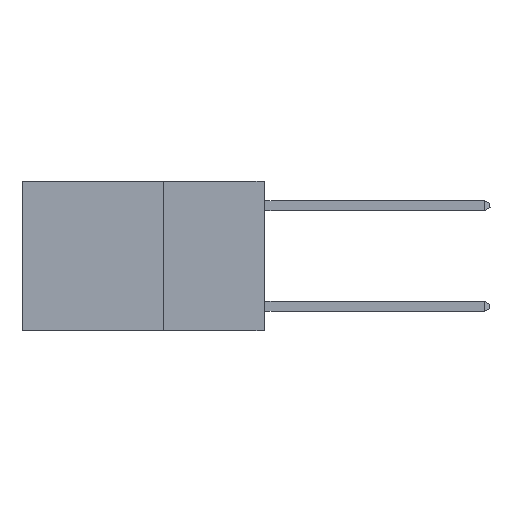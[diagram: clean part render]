
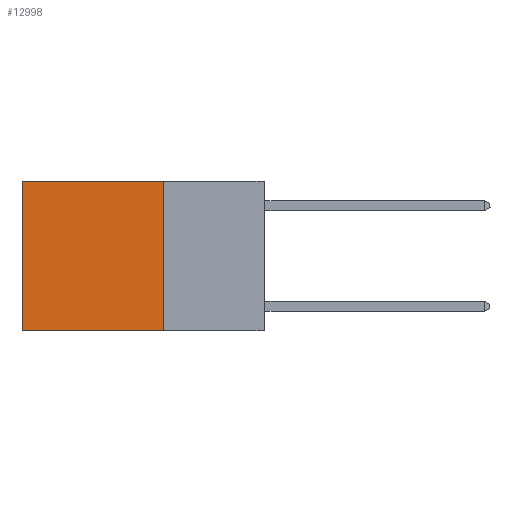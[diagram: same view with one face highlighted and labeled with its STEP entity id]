
A CAD part, left-side view. The second image highlights one B-rep face of the part: STEP entity #12998.
In plain terms, the highlighted planar face has unit normal (-1, 0, 0).
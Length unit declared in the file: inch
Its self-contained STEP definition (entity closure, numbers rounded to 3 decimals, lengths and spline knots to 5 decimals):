
#465 = PLANE ( 'NONE',  #9462 ) ;
#711 = ORIENTED_EDGE ( 'NONE', *, *, #20287, .T. ) ;
#3933 = DIRECTION ( 'NONE',  ( 0., 0., -1. ) ) ;
#4129 = DIRECTION ( 'NONE',  ( 0., 1., 0. ) ) ;
#4646 = FACE_OUTER_BOUND ( 'NONE', #7183, .T. ) ;
#4830 = EDGE_CURVE ( 'NONE', #15599, #10768, #7219, .T. ) ;
#6835 = DIRECTION ( 'NONE',  ( 0., 0., -1. ) ) ;
#7183 = EDGE_LOOP ( 'NONE', ( #711, #16482, #10879, #25299 ) ) ;
#7219 = LINE ( 'NONE', #8785, #12250 ) ;
#7361 = LINE ( 'NONE', #23371, #24555 ) ;
#8785 = CARTESIAN_POINT ( 'NONE',  ( 0.2625, 0.25, -0.37 ) ) ;
#9462 = AXIS2_PLACEMENT_3D ( 'NONE', #24105, #13250, #6835 ) ;
#10336 = VECTOR ( 'NONE', #12758, 39.37008 ) ;
#10722 = CARTESIAN_POINT ( 'NONE',  ( 0.2625, 0.25, -0.37 ) ) ;
#10768 = VERTEX_POINT ( 'NONE', #11291 ) ;
#10879 = ORIENTED_EDGE ( 'NONE', *, *, #14255, .F. ) ;
#11291 = CARTESIAN_POINT ( 'NONE',  ( 0.2625, 0.6, -0.37 ) ) ;
#12080 = VERTEX_POINT ( 'NONE', #22769 ) ;
#12143 = DIRECTION ( 'NONE',  ( 0., 1., 0. ) ) ;
#12250 = VECTOR ( 'NONE', #4129, 39.37008 ) ;
#12266 = CARTESIAN_POINT ( 'NONE',  ( 0.2625, 0.25, 0. ) ) ;
#12687 = VECTOR ( 'NONE', #3933, 39.37008 ) ;
#12758 = DIRECTION ( 'NONE',  ( 0., 0., -1. ) ) ;
#12998 = ADVANCED_FACE ( 'NONE', ( #4646 ), #465, .F. ) ;
#13250 = DIRECTION ( 'NONE',  ( 1., 0., 0. ) ) ;
#14255 = EDGE_CURVE ( 'NONE', #12080, #15599, #16061, .T. ) ;
#14882 = VERTEX_POINT ( 'NONE', #18795 ) ;
#15599 = VERTEX_POINT ( 'NONE', #10722 ) ;
#16061 = LINE ( 'NONE', #12266, #12687 ) ;
#16482 = ORIENTED_EDGE ( 'NONE', *, *, #4830, .F. ) ;
#17452 = CARTESIAN_POINT ( 'NONE',  ( 0.2625, 0.6, 0. ) ) ;
#18795 = CARTESIAN_POINT ( 'NONE',  ( 0.2625, 0.6, 0. ) ) ;
#19486 = EDGE_CURVE ( 'NONE', #12080, #14882, #7361, .T. ) ;
#20287 = EDGE_CURVE ( 'NONE', #14882, #10768, #27200, .T. ) ;
#22769 = CARTESIAN_POINT ( 'NONE',  ( 0.2625, 0.25, 0. ) ) ;
#23371 = CARTESIAN_POINT ( 'NONE',  ( 0.2625, 0.25, 0. ) ) ;
#24105 = CARTESIAN_POINT ( 'NONE',  ( 0.2625, 0.25, 0. ) ) ;
#24555 = VECTOR ( 'NONE', #12143, 39.37008 ) ;
#25299 = ORIENTED_EDGE ( 'NONE', *, *, #19486, .T. ) ;
#27200 = LINE ( 'NONE', #17452, #10336 ) ;
